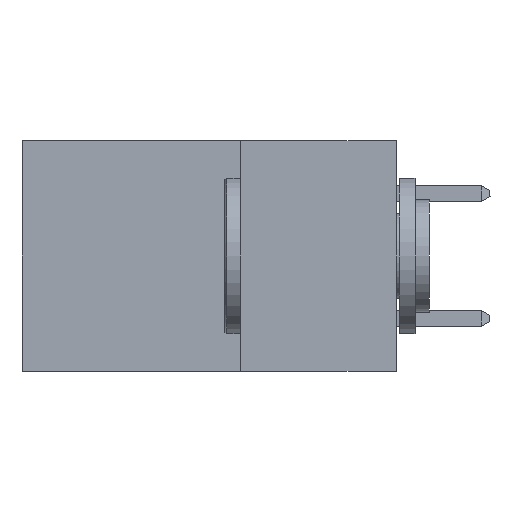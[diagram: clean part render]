
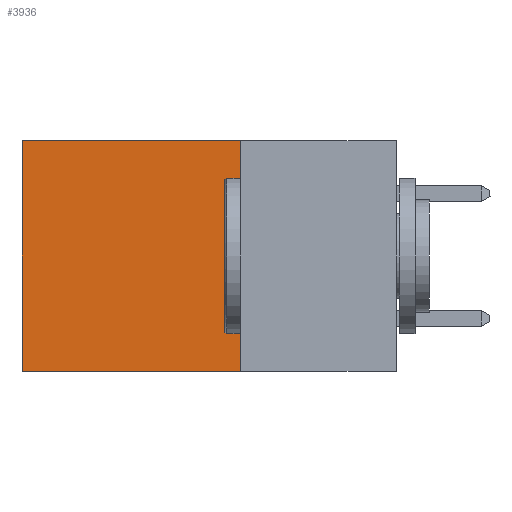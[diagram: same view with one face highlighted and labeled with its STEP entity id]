
A CAD part, left-side view. The second image highlights one B-rep face of the part: STEP entity #3936.
In plain terms, the highlighted planar face has unit normal (-1, 0, 0).
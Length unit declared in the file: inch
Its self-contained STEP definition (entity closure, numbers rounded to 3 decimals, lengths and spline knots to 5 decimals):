
#450 = ORIENTED_EDGE ( 'NONE', *, *, #23577, .F. ) ;
#485 = VECTOR ( 'NONE', #9707, 39.37008 ) ;
#488 = LINE ( 'NONE', #21604, #5298 ) ;
#1123 = LINE ( 'NONE', #17739, #485 ) ;
#2450 = VERTEX_POINT ( 'NONE', #20208 ) ;
#2898 = FACE_OUTER_BOUND ( 'NONE', #20103, .T. ) ;
#3006 = DIRECTION ( 'NONE',  ( 0., 0., -1. ) ) ;
#3750 = PLANE ( 'NONE',  #14300 ) ;
#3754 = VERTEX_POINT ( 'NONE', #7534 ) ;
#3936 = ADVANCED_FACE ( 'NONE', ( #2898 ), #3750, .F. ) ;
#5298 = VECTOR ( 'NONE', #15673, 39.37008 ) ;
#7215 = EDGE_CURVE ( 'NONE', #22144, #2450, #8363, .T. ) ;
#7276 = CARTESIAN_POINT ( 'NONE',  ( 0.298, 0.25, -0.37 ) ) ;
#7534 = CARTESIAN_POINT ( 'NONE',  ( 0.298, 0.6, 0. ) ) ;
#7581 = VERTEX_POINT ( 'NONE', #25390 ) ;
#8316 = CARTESIAN_POINT ( 'NONE',  ( 0.298, 0.25, -0.37 ) ) ;
#8363 = LINE ( 'NONE', #8316, #13070 ) ;
#8494 = VECTOR ( 'NONE', #3006, 39.37008 ) ;
#9707 = DIRECTION ( 'NONE',  ( 0., 1., 0. ) ) ;
#13048 = CARTESIAN_POINT ( 'NONE',  ( 0.298, 0.25, 0. ) ) ;
#13070 = VECTOR ( 'NONE', #24343, 39.37008 ) ;
#13849 = LINE ( 'NONE', #21145, #8494 ) ;
#14300 = AXIS2_PLACEMENT_3D ( 'NONE', #13048, #25278, #25250 ) ;
#15673 = DIRECTION ( 'NONE',  ( 0., 0., -1. ) ) ;
#17739 = CARTESIAN_POINT ( 'NONE',  ( 0.298, 0.25, 0. ) ) ;
#19431 = ORIENTED_EDGE ( 'NONE', *, *, #22900, .T. ) ;
#19604 = ORIENTED_EDGE ( 'NONE', *, *, #7215, .F. ) ;
#20103 = EDGE_LOOP ( 'NONE', ( #20246, #19604, #450, #19431 ) ) ;
#20208 = CARTESIAN_POINT ( 'NONE',  ( 0.298, 0.6, -0.37 ) ) ;
#20246 = ORIENTED_EDGE ( 'NONE', *, *, #22766, .T. ) ;
#21145 = CARTESIAN_POINT ( 'NONE',  ( 0.298, 0.6, 0. ) ) ;
#21604 = CARTESIAN_POINT ( 'NONE',  ( 0.298, 0.25, 0. ) ) ;
#22144 = VERTEX_POINT ( 'NONE', #7276 ) ;
#22766 = EDGE_CURVE ( 'NONE', #3754, #2450, #13849, .T. ) ;
#22900 = EDGE_CURVE ( 'NONE', #7581, #3754, #1123, .T. ) ;
#23577 = EDGE_CURVE ( 'NONE', #7581, #22144, #488, .T. ) ;
#24343 = DIRECTION ( 'NONE',  ( 0., 1., 0. ) ) ;
#25250 = DIRECTION ( 'NONE',  ( 0., 0., -1. ) ) ;
#25278 = DIRECTION ( 'NONE',  ( 1., 0., 0. ) ) ;
#25390 = CARTESIAN_POINT ( 'NONE',  ( 0.298, 0.25, 0. ) ) ;
